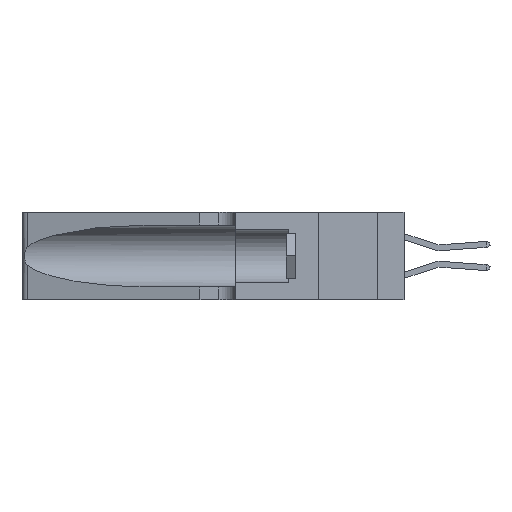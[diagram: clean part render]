
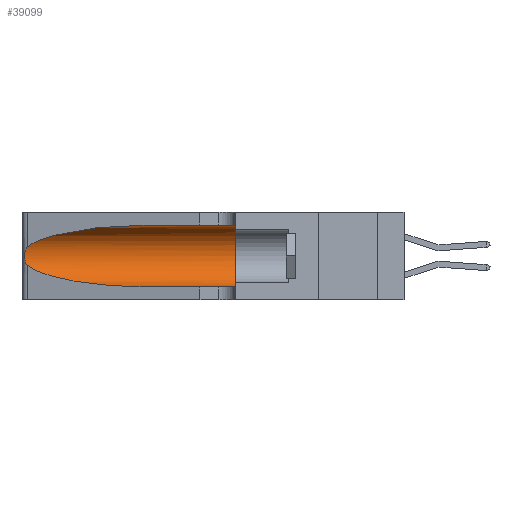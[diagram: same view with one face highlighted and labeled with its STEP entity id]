
A CAD part, left-side view. The second image highlights one B-rep face of the part: STEP entity #39099.
In plain terms, the highlighted cylindrical face has radius 3.308 mm (diameter 6.617 mm), a partial arc.
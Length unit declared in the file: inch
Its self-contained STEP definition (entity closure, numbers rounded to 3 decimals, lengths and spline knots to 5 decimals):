
#766 = CARTESIAN_POINT ( 'NONE',  ( 0.1305, 1.61858, 0.185 ) ) ;
#1982 = VERTEX_POINT ( 'NONE', #44011 ) ;
#2036 = AXIS2_PLACEMENT_3D ( 'NONE', #12665, #37742, #17100 ) ;
#2330 = ORIENTED_EDGE ( 'NONE', *, *, #10017, .F. ) ;
#2338 = CARTESIAN_POINT ( 'NONE',  ( 0.1305, 1.61858, 0.31525 ) ) ;
#2419 = EDGE_LOOP ( 'NONE', ( #29341, #42327, #37444, #20615, #18523, #2330 ) ) ;
#2947 = DIRECTION ( 'NONE',  ( 0., -1., 0. ) ) ;
#3264 = CARTESIAN_POINT ( 'NONE',  ( 0.1305, 1.61858, 0.05475 ) ) ;
#4937 = CARTESIAN_POINT ( 'NONE',  ( 0.25487, 1.22718, 0.22369 ) ) ;
#4968 = VERTEX_POINT ( 'NONE', #30491 ) ;
#5666 = VERTEX_POINT ( 'NONE', #9681 ) ;
#6660 = CARTESIAN_POINT ( 'NONE',  ( 0.25487, 1.22718, 0.14631 ) ) ;
#7864 = CARTESIAN_POINT ( 'NONE',  ( 0.25856, 1.23593, 0.16098 ) ) ;
#8298 = CARTESIAN_POINT ( 'NONE',  ( 0.1305, 0.72297, 0.31525 ) ) ;
#8530 = VECTOR ( 'NONE', #23559, 39.37008 ) ;
#9681 = CARTESIAN_POINT ( 'NONE',  ( 0.1305, 0.35, 0.05475 ) ) ;
#10017 = EDGE_CURVE ( 'NONE', #32995, #11709, #32499, .T. ) ;
#10184 = CARTESIAN_POINT ( 'NONE',  ( 0.2373, 1.15595, 0.08982 ) ) ;
#11227 = CARTESIAN_POINT ( 'NONE',  ( 0.26018, 1.23835, 0.19895 ) ) ;
#11528 = CARTESIAN_POINT ( 'NONE',  ( 0.25854, 1.2359, 0.20912 ) ) ;
#11709 = VERTEX_POINT ( 'NONE', #14304 ) ;
#11964 = VERTEX_POINT ( 'NONE', #20528 ) ;
#12059 =( BOUNDED_CURVE ( )  B_SPLINE_CURVE ( 3, ( #6660, #10184, #27978, #28271 ),
 .UNSPECIFIED., .F., .F. ) 
 B_SPLINE_CURVE_WITH_KNOTS ( ( 4, 4 ),
 ( 3.44316, 4.71239 ),
 .UNSPECIFIED. ) 
 CURVE ( )  GEOMETRIC_REPRESENTATION_ITEM ( )  RATIONAL_B_SPLINE_CURVE ( ( 1., 0.87, 0.87, 1. ) ) 
 REPRESENTATION_ITEM ( '' )  );
#12110 = VECTOR ( 'NONE', #2947, 39.37008 ) ;
#12665 = CARTESIAN_POINT ( 'NONE',  ( 0.1305, 0.35, 0.185 ) ) ;
#13209 = EDGE_CURVE ( 'NONE', #32995, #1982, #20152, .T. ) ;
#14018 = EDGE_CURVE ( 'NONE', #11709, #5666, #34355, .T. ) ;
#14304 = CARTESIAN_POINT ( 'NONE',  ( 0.1305, 0.35, 0.31525 ) ) ;
#14573 = CARTESIAN_POINT ( 'NONE',  ( 0.25487, 1.22718, 0.22369 ) ) ;
#14727 = CARTESIAN_POINT ( 'NONE',  ( 0.26075, 1.23896, 0.19203 ) ) ;
#17100 = DIRECTION ( 'NONE',  ( 0., 0., 1. ) ) ;
#17467 = EDGE_CURVE ( 'NONE', #4968, #11964, #12059, .T. ) ;
#18256 = CARTESIAN_POINT ( 'NONE',  ( 0.25555, 1.22994, 0.2215 ) ) ;
#18523 = ORIENTED_EDGE ( 'NONE', *, *, #14018, .F. ) ;
#18558 = CARTESIAN_POINT ( 'NONE',  ( 0.25487, 1.22718, 0.14631 ) ) ;
#20152 =( BOUNDED_CURVE ( )  B_SPLINE_CURVE ( 3, ( #25806, #32949, #22009, #4937 ),
 .UNSPECIFIED., .F., .T. ) 
 B_SPLINE_CURVE_WITH_KNOTS ( ( 4, 4 ),
 ( 1.5708, 2.84003 ),
 .UNSPECIFIED. ) 
 CURVE ( )  GEOMETRIC_REPRESENTATION_ITEM ( )  RATIONAL_B_SPLINE_CURVE ( ( 1., 0.87, 0.87, 1. ) ) 
 REPRESENTATION_ITEM ( '' )  );
#20528 = CARTESIAN_POINT ( 'NONE',  ( 0.1305, 0.72297, 0.05475 ) ) ;
#20615 = ORIENTED_EDGE ( 'NONE', *, *, #31038, .T. ) ;
#21878 = CARTESIAN_POINT ( 'NONE',  ( 0.25787, 1.23484, 0.2124 ) ) ;
#22009 = CARTESIAN_POINT ( 'NONE',  ( 0.2373, 1.15595, 0.28018 ) ) ;
#23559 = DIRECTION ( 'NONE',  ( 0., -1., 0. ) ) ;
#25015 = DIRECTION ( 'NONE',  ( 0., 0., -1. ) ) ;
#25213 = CARTESIAN_POINT ( 'NONE',  ( 0.26017, 1.23833, 0.17102 ) ) ;
#25510 = CARTESIAN_POINT ( 'NONE',  ( 0.25639, 1.23184, 0.21858 ) ) ;
#25806 = CARTESIAN_POINT ( 'NONE',  ( 0.1305, 0.72297, 0.31525 ) ) ;
#27559 = AXIS2_PLACEMENT_3D ( 'NONE', #766, #35054, #25015 ) ;
#27978 = CARTESIAN_POINT ( 'NONE',  ( 0.18966, 0.96281, 0.05475 ) ) ;
#28271 = CARTESIAN_POINT ( 'NONE',  ( 0.1305, 0.72297, 0.05475 ) ) ;
#29016 = CARTESIAN_POINT ( 'NONE',  ( 0.26075, 1.23896, 0.178 ) ) ;
#29341 = ORIENTED_EDGE ( 'NONE', *, *, #13209, .T. ) ;
#30491 = CARTESIAN_POINT ( 'NONE',  ( 0.25487, 1.22718, 0.14631 ) ) ;
#31038 = EDGE_CURVE ( 'NONE', #11964, #5666, #35473, .T. ) ;
#32210 = CARTESIAN_POINT ( 'NONE',  ( 0.25639, 1.23186, 0.15144 ) ) ;
#32499 = LINE ( 'NONE', #2338, #8530 ) ;
#32949 = CARTESIAN_POINT ( 'NONE',  ( 0.18966, 0.96281, 0.31525 ) ) ;
#32995 = VERTEX_POINT ( 'NONE', #8298 ) ;
#34355 = CIRCLE ( 'NONE', #2036, 0.13025 ) ;
#35054 = DIRECTION ( 'NONE',  ( 0., -1., 0. ) ) ;
#35473 = LINE ( 'NONE', #3264, #12110 ) ;
#37444 = ORIENTED_EDGE ( 'NONE', *, *, #17467, .T. ) ;
#37742 = DIRECTION ( 'NONE',  ( 0., 1., 0. ) ) ;
#38529 = CYLINDRICAL_SURFACE ( 'NONE', #27559, 0.13025 ) ;
#38899 = CARTESIAN_POINT ( 'NONE',  ( 0.25789, 1.23486, 0.15765 ) ) ;
#39099 = ADVANCED_FACE ( 'NONE', ( #40734 ), #38529, .F. ) ;
#39359 = CARTESIAN_POINT ( 'NONE',  ( 0.25555, 1.22993, 0.14849 ) ) ;
#39920 = B_SPLINE_CURVE_WITH_KNOTS ( 'NONE', 3,
 ( #14573, #18256, #25510, #21878, #11528, #11227, #14727, #29016, #25213, #7864, #38899, #32210, #39359, #18558 ),
 .UNSPECIFIED., .F., .F.,
 ( 4, 2, 2, 2, 2, 2, 4 ),
 ( 0., 0.00027, 0.00053, 0.00107, 0.0016, 0.00187, 0.00214 ),
 .UNSPECIFIED. ) ;
#40734 = FACE_OUTER_BOUND ( 'NONE', #2419, .T. ) ;
#42327 = ORIENTED_EDGE ( 'NONE', *, *, #44156, .T. ) ;
#44011 = CARTESIAN_POINT ( 'NONE',  ( 0.25487, 1.22718, 0.22369 ) ) ;
#44156 = EDGE_CURVE ( 'NONE', #1982, #4968, #39920, .T. ) ;
